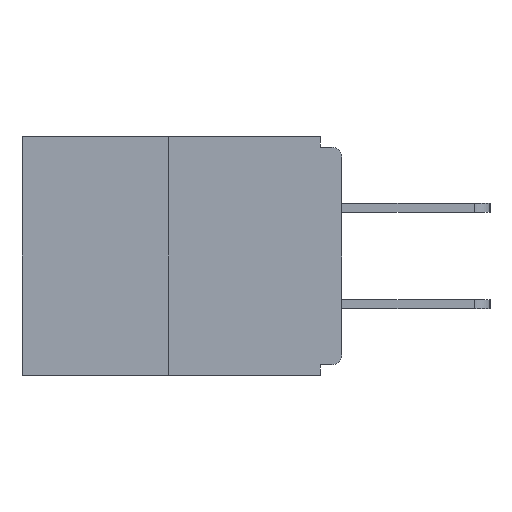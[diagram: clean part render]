
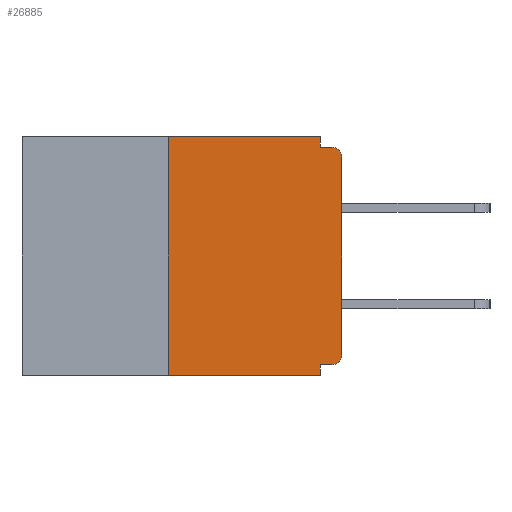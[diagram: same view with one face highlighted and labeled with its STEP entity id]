
A CAD part, left-side view. The second image highlights one B-rep face of the part: STEP entity #26885.
In plain terms, the highlighted planar face has unit normal (-1, 0, 0).
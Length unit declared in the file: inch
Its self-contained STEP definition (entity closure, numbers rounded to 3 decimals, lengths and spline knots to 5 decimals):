
#154 = CARTESIAN_POINT ( 'NONE',  ( 0., 0., 0. ) ) ;
#324 = ORIENTED_EDGE ( 'NONE', *, *, #29942, .T. ) ;
#884 = DIRECTION ( 'NONE',  ( 0., -1., 0. ) ) ;
#911 = VECTOR ( 'NONE', #3286, 39.37008 ) ;
#999 = CARTESIAN_POINT ( 'NONE',  ( 0., 0.46, -0.343 ) ) ;
#1015 = VERTEX_POINT ( 'NONE', #2037 ) ;
#1016 = LINE ( 'NONE', #24389, #24952 ) ;
#1202 = DIRECTION ( 'NONE',  ( 0., -1., 0. ) ) ;
#1928 = CARTESIAN_POINT ( 'NONE',  ( 0., 0., -0.313 ) ) ;
#2037 = CARTESIAN_POINT ( 'NONE',  ( 0., 0.031, -0.015 ) ) ;
#2699 = EDGE_LOOP ( 'NONE', ( #22053, #19097, #28759, #24655, #10329, #6104, #324, #10580, #16244, #9631 ) ) ;
#2937 = VECTOR ( 'NONE', #28565, 39.37008 ) ;
#3007 = VECTOR ( 'NONE', #1202, 39.37008 ) ;
#3286 = DIRECTION ( 'NONE',  ( 0., 0., 1. ) ) ;
#3432 = AXIS2_PLACEMENT_3D ( 'NONE', #13493, #25153, #9103 ) ;
#3913 = LINE ( 'NONE', #11675, #18415 ) ;
#4757 = CIRCLE ( 'NONE', #3432, 0.015 ) ;
#5259 = VERTEX_POINT ( 'NONE', #1928 ) ;
#5301 = VECTOR ( 'NONE', #884, 39.37008 ) ;
#5352 = PLANE ( 'NONE',  #29083 ) ;
#5771 = VECTOR ( 'NONE', #11969, 39.37008 ) ;
#6073 = DIRECTION ( 'NONE',  ( 0., 0., -1. ) ) ;
#6104 = ORIENTED_EDGE ( 'NONE', *, *, #24937, .T. ) ;
#6186 = CARTESIAN_POINT ( 'NONE',  ( 0., 0.25, 0. ) ) ;
#7663 = CARTESIAN_POINT ( 'NONE',  ( 0., 0.46, 0. ) ) ;
#7748 = VERTEX_POINT ( 'NONE', #13950 ) ;
#7932 = LINE ( 'NONE', #154, #5771 ) ;
#8645 = DIRECTION ( 'NONE',  ( -1., 0., 0. ) ) ;
#8746 = DIRECTION ( 'NONE',  ( 0., 1., 0. ) ) ;
#9103 = DIRECTION ( 'NONE',  ( 0., 0., -1. ) ) ;
#9631 = ORIENTED_EDGE ( 'NONE', *, *, #12542, .F. ) ;
#10329 = ORIENTED_EDGE ( 'NONE', *, *, #10405, .F. ) ;
#10387 = CARTESIAN_POINT ( 'NONE',  ( 0., 0.031, -0.343 ) ) ;
#10405 = EDGE_CURVE ( 'NONE', #29613, #10925, #12313, .T. ) ;
#10580 = ORIENTED_EDGE ( 'NONE', *, *, #27139, .T. ) ;
#10621 = DIRECTION ( 'NONE',  ( 1., 0., 0. ) ) ;
#10913 = LINE ( 'NONE', #10387, #2937 ) ;
#10925 = VERTEX_POINT ( 'NONE', #17947 ) ;
#11298 = DIRECTION ( 'NONE',  ( 0., -1., 0. ) ) ;
#11675 = CARTESIAN_POINT ( 'NONE',  ( 0., 0., -0.015 ) ) ;
#11735 = EDGE_CURVE ( 'NONE', #1015, #17789, #3913, .T. ) ;
#11969 = DIRECTION ( 'NONE',  ( 0., 0., 1. ) ) ;
#12207 = LINE ( 'NONE', #21106, #5301 ) ;
#12313 = LINE ( 'NONE', #27510, #13069 ) ;
#12542 = EDGE_CURVE ( 'NONE', #25114, #1015, #1016, .T. ) ;
#12920 = DIRECTION ( 'NONE',  ( 0., 0., -1. ) ) ;
#12966 = CARTESIAN_POINT ( 'NONE',  ( 0., 0.031, -0.343 ) ) ;
#13069 = VECTOR ( 'NONE', #8746, 39.37008 ) ;
#13493 = CARTESIAN_POINT ( 'NONE',  ( 0., 0.015, -0.313 ) ) ;
#13950 = CARTESIAN_POINT ( 'NONE',  ( 0., 0., -0.03 ) ) ;
#14617 = AXIS2_PLACEMENT_3D ( 'NONE', #26704, #8645, #24902 ) ;
#15073 = EDGE_CURVE ( 'NONE', #25335, #23650, #24775, .T. ) ;
#16244 = ORIENTED_EDGE ( 'NONE', *, *, #11735, .F. ) ;
#16858 = EDGE_CURVE ( 'NONE', #17155, #25114, #12207, .T. ) ;
#17155 = VERTEX_POINT ( 'NONE', #6186 ) ;
#17789 = VERTEX_POINT ( 'NONE', #28419 ) ;
#17907 = CARTESIAN_POINT ( 'NONE',  ( 0., 0.25, -0.343 ) ) ;
#17947 = CARTESIAN_POINT ( 'NONE',  ( 0., 0.031, -0.328 ) ) ;
#18400 = CIRCLE ( 'NONE', #14617, 0.015 ) ;
#18415 = VECTOR ( 'NONE', #11298, 39.37008 ) ;
#18989 = CARTESIAN_POINT ( 'NONE',  ( 0., 0.031, 0. ) ) ;
#19097 = ORIENTED_EDGE ( 'NONE', *, *, #23071, .F. ) ;
#19362 = LINE ( 'NONE', #29129, #911 ) ;
#20722 = EDGE_CURVE ( 'NONE', #10925, #23650, #10913, .T. ) ;
#21106 = CARTESIAN_POINT ( 'NONE',  ( 0., 0.46, 0. ) ) ;
#22053 = ORIENTED_EDGE ( 'NONE', *, *, #16858, .F. ) ;
#23071 = EDGE_CURVE ( 'NONE', #25335, #17155, #19362, .T. ) ;
#23650 = VERTEX_POINT ( 'NONE', #12966 ) ;
#24389 = CARTESIAN_POINT ( 'NONE',  ( 0., 0.031, 0. ) ) ;
#24655 = ORIENTED_EDGE ( 'NONE', *, *, #20722, .F. ) ;
#24775 = LINE ( 'NONE', #999, #3007 ) ;
#24902 = DIRECTION ( 'NONE',  ( 0., 0., -1. ) ) ;
#24937 = EDGE_CURVE ( 'NONE', #29613, #5259, #4757, .T. ) ;
#24952 = VECTOR ( 'NONE', #12920, 39.37008 ) ;
#25114 = VERTEX_POINT ( 'NONE', #18989 ) ;
#25153 = DIRECTION ( 'NONE',  ( -1., 0., 0. ) ) ;
#25335 = VERTEX_POINT ( 'NONE', #17907 ) ;
#26704 = CARTESIAN_POINT ( 'NONE',  ( 0., 0.015, -0.03 ) ) ;
#26885 = ADVANCED_FACE ( 'NONE', ( #28914 ), #5352, .F. ) ;
#27139 = EDGE_CURVE ( 'NONE', #7748, #17789, #18400, .T. ) ;
#27510 = CARTESIAN_POINT ( 'NONE',  ( 0., 0., -0.328 ) ) ;
#28419 = CARTESIAN_POINT ( 'NONE',  ( 0., 0.015, -0.015 ) ) ;
#28545 = CARTESIAN_POINT ( 'NONE',  ( 0., 0.015, -0.328 ) ) ;
#28565 = DIRECTION ( 'NONE',  ( 0., 0., -1. ) ) ;
#28759 = ORIENTED_EDGE ( 'NONE', *, *, #15073, .T. ) ;
#28914 = FACE_OUTER_BOUND ( 'NONE', #2699, .T. ) ;
#29083 = AXIS2_PLACEMENT_3D ( 'NONE', #7663, #10621, #6073 ) ;
#29129 = CARTESIAN_POINT ( 'NONE',  ( 0., 0.25, 0. ) ) ;
#29613 = VERTEX_POINT ( 'NONE', #28545 ) ;
#29942 = EDGE_CURVE ( 'NONE', #5259, #7748, #7932, .T. ) ;
